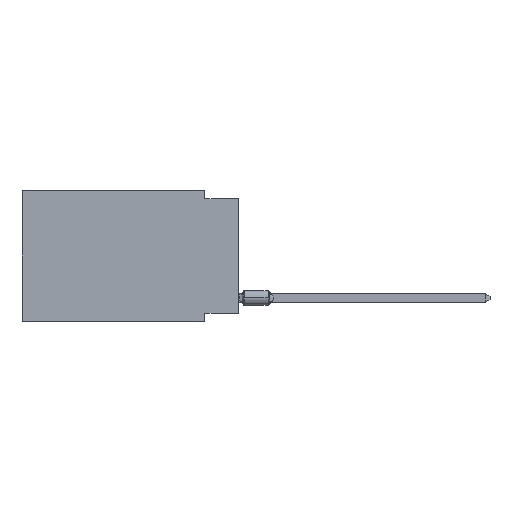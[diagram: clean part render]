
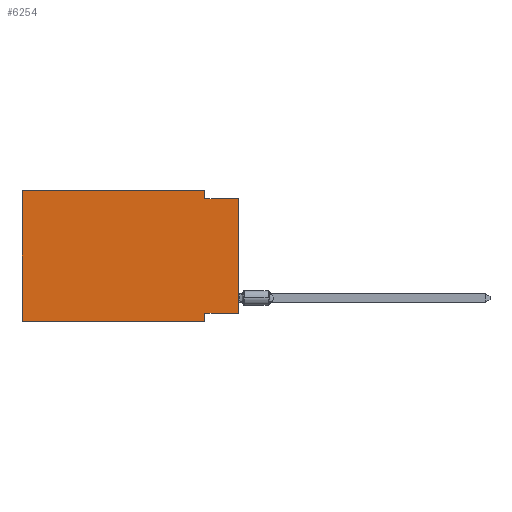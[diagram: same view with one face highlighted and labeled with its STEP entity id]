
A CAD part, left-side view. The second image highlights one B-rep face of the part: STEP entity #6254.
In plain terms, the highlighted planar face has unit normal (-1, 0, 0).
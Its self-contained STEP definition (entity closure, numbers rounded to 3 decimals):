
#100 = DIRECTION ( 'NONE',  ( 0., 0., -1. ) ) ;
#140 = VERTEX_POINT ( 'NONE', #10222 ) ;
#335 = CARTESIAN_POINT ( 'NONE',  ( 0., 2.54, -9.906 ) ) ;
#1232 = EDGE_CURVE ( 'NONE', #5383, #2875, #23445, .T. ) ;
#1453 = CARTESIAN_POINT ( 'NONE',  ( 0., 16.383, 0. ) ) ;
#1612 = CARTESIAN_POINT ( 'NONE',  ( 0., 0., -9.271 ) ) ;
#1749 = VECTOR ( 'NONE', #17499, 1000. ) ;
#2875 = VERTEX_POINT ( 'NONE', #4620 ) ;
#3437 = ORIENTED_EDGE ( 'NONE', *, *, #1232, .F. ) ;
#4536 = ORIENTED_EDGE ( 'NONE', *, *, #11590, .F. ) ;
#4620 = CARTESIAN_POINT ( 'NONE',  ( 0., 2.54, 0. ) ) ;
#4751 = CARTESIAN_POINT ( 'NONE',  ( 0., 16.383, 0. ) ) ;
#4776 = VECTOR ( 'NONE', #27674, 1000. ) ;
#4859 = ORIENTED_EDGE ( 'NONE', *, *, #11439, .F. ) ;
#5111 = DIRECTION ( 'NONE',  ( 0., 0., -1. ) ) ;
#5383 = VERTEX_POINT ( 'NONE', #8370 ) ;
#5635 = CARTESIAN_POINT ( 'NONE',  ( 0., 0., 0. ) ) ;
#6254 = ADVANCED_FACE ( 'NONE', ( #19951 ), #21643, .F. ) ;
#7886 = VERTEX_POINT ( 'NONE', #335 ) ;
#8274 = AXIS2_PLACEMENT_3D ( 'NONE', #4751, #26154, #100 ) ;
#8370 = CARTESIAN_POINT ( 'NONE',  ( 0., 16.383, 0. ) ) ;
#8783 = CARTESIAN_POINT ( 'NONE',  ( 0., 16.383, -9.906 ) ) ;
#9083 = ORIENTED_EDGE ( 'NONE', *, *, #15087, .T. ) ;
#9537 = EDGE_CURVE ( 'NONE', #2875, #140, #22082, .T. ) ;
#10222 = CARTESIAN_POINT ( 'NONE',  ( 0., 2.54, -0.635 ) ) ;
#10308 = VERTEX_POINT ( 'NONE', #8783 ) ;
#11439 = EDGE_CURVE ( 'NONE', #140, #19540, #26113, .T. ) ;
#11590 = EDGE_CURVE ( 'NONE', #10308, #5383, #14250, .T. ) ;
#13066 = VERTEX_POINT ( 'NONE', #25678 ) ;
#13477 = EDGE_CURVE ( 'NONE', #10308, #7886, #14369, .T. ) ;
#14211 = DIRECTION ( 'NONE',  ( 0., 0., 1. ) ) ;
#14250 = LINE ( 'NONE', #1453, #24701 ) ;
#14369 = LINE ( 'NONE', #22828, #17133 ) ;
#14584 = EDGE_LOOP ( 'NONE', ( #9083, #4859, #22661, #3437, #4536, #17323, #26373, #21149 ) ) ;
#15087 = EDGE_CURVE ( 'NONE', #13066, #19540, #25203, .T. ) ;
#17133 = VECTOR ( 'NONE', #22974, 1000. ) ;
#17323 = ORIENTED_EDGE ( 'NONE', *, *, #13477, .T. ) ;
#17499 = DIRECTION ( 'NONE',  ( 0., -1., 0. ) ) ;
#18338 = VECTOR ( 'NONE', #14211, 1000. ) ;
#18777 = LINE ( 'NONE', #1612, #18883 ) ;
#18883 = VECTOR ( 'NONE', #23168, 1000. ) ;
#19540 = VERTEX_POINT ( 'NONE', #21622 ) ;
#19621 = CARTESIAN_POINT ( 'NONE',  ( 0., 0., -0.635 ) ) ;
#19951 = FACE_OUTER_BOUND ( 'NONE', #14584, .T. ) ;
#20083 = EDGE_CURVE ( 'NONE', #27562, #7886, #20444, .T. ) ;
#20103 = CARTESIAN_POINT ( 'NONE',  ( 0., 2.54, 0. ) ) ;
#20389 = VECTOR ( 'NONE', #5111, 1000. ) ;
#20444 = LINE ( 'NONE', #24662, #20389 ) ;
#20783 = CARTESIAN_POINT ( 'NONE',  ( 0., 16.383, 0. ) ) ;
#20809 = CARTESIAN_POINT ( 'NONE',  ( 0., 2.54, -9.271 ) ) ;
#21131 = EDGE_CURVE ( 'NONE', #13066, #27562, #18777, .T. ) ;
#21149 = ORIENTED_EDGE ( 'NONE', *, *, #21131, .F. ) ;
#21622 = CARTESIAN_POINT ( 'NONE',  ( 0., 0., -0.635 ) ) ;
#21643 = PLANE ( 'NONE',  #8274 ) ;
#22082 = LINE ( 'NONE', #20103, #25091 ) ;
#22661 = ORIENTED_EDGE ( 'NONE', *, *, #9537, .F. ) ;
#22828 = CARTESIAN_POINT ( 'NONE',  ( 0., 16.383, -9.906 ) ) ;
#22974 = DIRECTION ( 'NONE',  ( 0., -1., 0. ) ) ;
#23168 = DIRECTION ( 'NONE',  ( 0., 1., 0. ) ) ;
#23445 = LINE ( 'NONE', #20783, #4776 ) ;
#24662 = CARTESIAN_POINT ( 'NONE',  ( 0., 2.54, -9.906 ) ) ;
#24701 = VECTOR ( 'NONE', #24835, 1000. ) ;
#24835 = DIRECTION ( 'NONE',  ( 0., 0., 1. ) ) ;
#25091 = VECTOR ( 'NONE', #26450, 1000. ) ;
#25203 = LINE ( 'NONE', #5635, #18338 ) ;
#25678 = CARTESIAN_POINT ( 'NONE',  ( 0., 0., -9.271 ) ) ;
#26113 = LINE ( 'NONE', #19621, #1749 ) ;
#26154 = DIRECTION ( 'NONE',  ( 1., 0., 0. ) ) ;
#26373 = ORIENTED_EDGE ( 'NONE', *, *, #20083, .F. ) ;
#26450 = DIRECTION ( 'NONE',  ( 0., 0., -1. ) ) ;
#27562 = VERTEX_POINT ( 'NONE', #20809 ) ;
#27674 = DIRECTION ( 'NONE',  ( 0., -1., 0. ) ) ;
